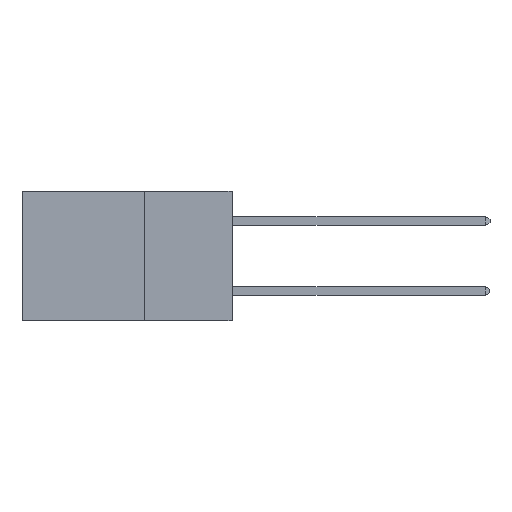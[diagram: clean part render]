
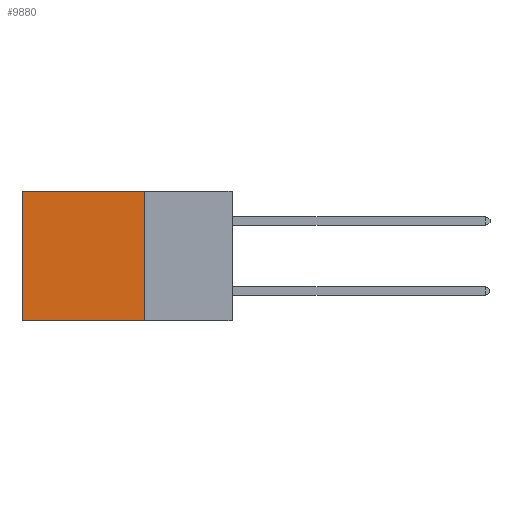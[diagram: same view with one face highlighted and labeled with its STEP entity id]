
A CAD part, left-side view. The second image highlights one B-rep face of the part: STEP entity #9880.
In plain terms, the highlighted planar face has unit normal (-1, 0, 0).
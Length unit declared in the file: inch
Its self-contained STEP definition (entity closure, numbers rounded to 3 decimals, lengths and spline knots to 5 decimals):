
#503 = CARTESIAN_POINT ( 'NONE',  ( 0.2875, 0.25, -0.37 ) ) ;
#715 = ORIENTED_EDGE ( 'NONE', *, *, #8930, .F. ) ;
#1771 = LINE ( 'NONE', #8508, #14636 ) ;
#2144 = VERTEX_POINT ( 'NONE', #503 ) ;
#3246 = ORIENTED_EDGE ( 'NONE', *, *, #4451, .F. ) ;
#3401 = CARTESIAN_POINT ( 'NONE',  ( 0.2875, 0.25, 0. ) ) ;
#4451 = EDGE_CURVE ( 'NONE', #2144, #14441, #14500, .T. ) ;
#4563 = LINE ( 'NONE', #7585, #14150 ) ;
#4667 = DIRECTION ( 'NONE',  ( 0., 0., -1. ) ) ;
#4792 = LINE ( 'NONE', #3401, #11194 ) ;
#5402 = PLANE ( 'NONE',  #9396 ) ;
#5459 = CARTESIAN_POINT ( 'NONE',  ( 0.2875, 0.25, 0. ) ) ;
#5512 = DIRECTION ( 'NONE',  ( 0., 0., -1. ) ) ;
#5850 = EDGE_CURVE ( 'NONE', #11234, #14441, #1771, .T. ) ;
#6869 = CARTESIAN_POINT ( 'NONE',  ( 0.2875, 0.6, -0.37 ) ) ;
#7585 = CARTESIAN_POINT ( 'NONE',  ( 0.2875, 0.25, 0. ) ) ;
#8508 = CARTESIAN_POINT ( 'NONE',  ( 0.2875, 0.6, 0. ) ) ;
#8930 = EDGE_CURVE ( 'NONE', #15418, #2144, #4792, .T. ) ;
#9396 = AXIS2_PLACEMENT_3D ( 'NONE', #5459, #13070, #5512 ) ;
#9859 = DIRECTION ( 'NONE',  ( 0., 1., 0. ) ) ;
#9880 = ADVANCED_FACE ( 'NONE', ( #11156 ), #5402, .F. ) ;
#10860 = ORIENTED_EDGE ( 'NONE', *, *, #5850, .T. ) ;
#11156 = FACE_OUTER_BOUND ( 'NONE', #14925, .T. ) ;
#11194 = VECTOR ( 'NONE', #4667, 39.37008 ) ;
#11234 = VERTEX_POINT ( 'NONE', #15348 ) ;
#12882 = CARTESIAN_POINT ( 'NONE',  ( 0.2875, 0.25, -0.37 ) ) ;
#13070 = DIRECTION ( 'NONE',  ( 1., 0., 0. ) ) ;
#13550 = DIRECTION ( 'NONE',  ( 0., 0., -1. ) ) ;
#14134 = VECTOR ( 'NONE', #9859, 39.37008 ) ;
#14150 = VECTOR ( 'NONE', #14971, 39.37008 ) ;
#14204 = EDGE_CURVE ( 'NONE', #15418, #11234, #4563, .T. ) ;
#14394 = ORIENTED_EDGE ( 'NONE', *, *, #14204, .T. ) ;
#14441 = VERTEX_POINT ( 'NONE', #6869 ) ;
#14500 = LINE ( 'NONE', #12882, #14134 ) ;
#14636 = VECTOR ( 'NONE', #13550, 39.37008 ) ;
#14925 = EDGE_LOOP ( 'NONE', ( #10860, #3246, #715, #14394 ) ) ;
#14971 = DIRECTION ( 'NONE',  ( 0., 1., 0. ) ) ;
#15348 = CARTESIAN_POINT ( 'NONE',  ( 0.2875, 0.6, 0. ) ) ;
#15418 = VERTEX_POINT ( 'NONE', #16031 ) ;
#16031 = CARTESIAN_POINT ( 'NONE',  ( 0.2875, 0.25, 0. ) ) ;
